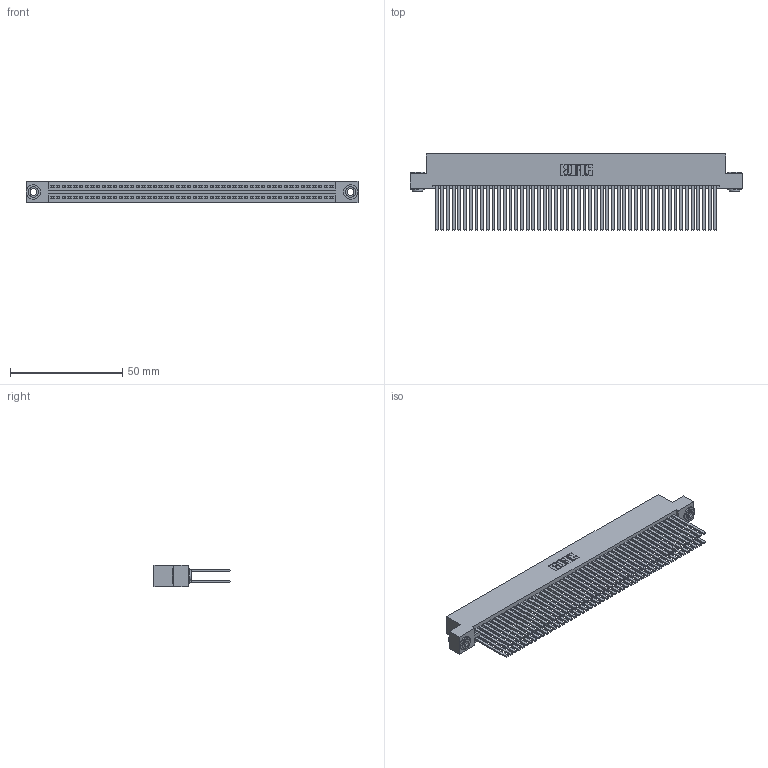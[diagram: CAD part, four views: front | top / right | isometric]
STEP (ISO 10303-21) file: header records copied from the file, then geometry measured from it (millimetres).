
FILE_DESCRIPTION (( 'STEP AP203' ), '1' );
FILE_NAME ('345-100-544-203.STEP', '2018-10-05T15:46:05', ( '' ), ( '' ), 'SwSTEP 2.0', 'SolidWorks 2016', '' );
FILE_SCHEMA (( 'CONFIG_CONTROL_DESIGN' ));
Length unit declared in the file: inch
Products named in the file (4): 345 Part_Flush Mounting Lugs - 0.156 Dia-TH; 345-250-002_345-250-002-102; 345-100-544-203; 345-292-001_345-293-144
Assembly tree (103 placements, depth 2):
  345-100-544-203
    345 Part_Flush Mounting Lugs - 0.156 Dia-TH
    345-292-001_345-293-144  x100
    345-250-002_345-250-002-102  x2
Bounding box: 148.21 x 33.96 x 9.4 mm (x, y, z)
Volume: 15892.6 mm3; surface area: 27960.4 mm2
Topology: 103 solids, 103 shells, 4564 faces, 13517 edges, 8874 vertices
Faces by surface type: plane 2990, cylinder 1566, cone 8
Entity records: 38620 total; most frequent: CARTESIAN_POINT 6439, ORIENTED_EDGE 6366, DIRECTION 5697, EDGE_CURVE 3183, VECTOR 2831, LINE 2831, VERTEX_POINT 2118, AXIS2_PLACEMENT_3D 1433
